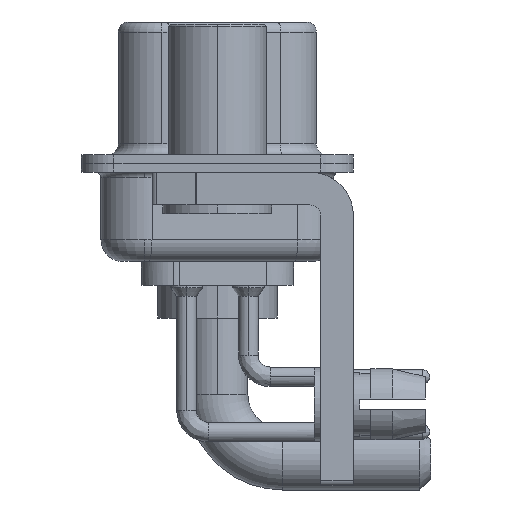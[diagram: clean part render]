
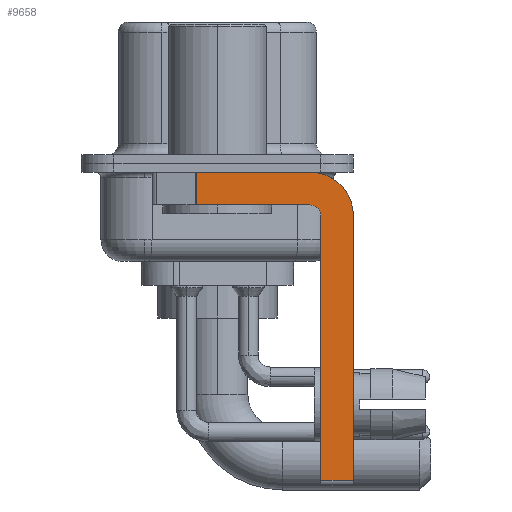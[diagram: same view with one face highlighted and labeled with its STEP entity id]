
A CAD part, left-side view. The second image highlights one B-rep face of the part: STEP entity #9658.
In plain terms, the highlighted planar face has unit normal (-1, 0, 0).
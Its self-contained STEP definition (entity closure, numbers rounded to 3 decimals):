
#695 = EDGE_LOOP ( 'NONE', ( #3606, #11332, #12984, #16502, #7405, #11200, #17029, #29080 ) ) ;
#768 = EDGE_CURVE ( 'NONE', #21767, #13116, #26312, .T. ) ;
#814 = DIRECTION ( 'NONE',  ( 0., 0., 1. ) ) ;
#1452 = VECTOR ( 'NONE', #12609, 1000. ) ;
#1464 = CARTESIAN_POINT ( 'NONE',  ( -2.9, 3., -0.4 ) ) ;
#2760 = DIRECTION ( 'NONE',  ( -1., 0., 0. ) ) ;
#2823 = CARTESIAN_POINT ( 'NONE',  ( -2.9, -4.25, -1.9 ) ) ;
#3297 = CARTESIAN_POINT ( 'NONE',  ( -2.9, 0.978, -1.9 ) ) ;
#3606 = ORIENTED_EDGE ( 'NONE', *, *, #768, .F. ) ;
#4051 = CIRCLE ( 'NONE', #5938, 2. ) ;
#4072 = CARTESIAN_POINT ( 'NONE',  ( -2.9, -4.75, -14.55 ) ) ;
#4102 = CARTESIAN_POINT ( 'NONE',  ( -2.9, -4.75, -14.8 ) ) ;
#4115 = EDGE_CURVE ( 'NONE', #13116, #25936, #4051, .T. ) ;
#4164 = EDGE_CURVE ( 'NONE', #28870, #18369, #13139, .T. ) ;
#4523 = CARTESIAN_POINT ( 'NONE',  ( -2.9, -4.25, -14.55 ) ) ;
#5938 = AXIS2_PLACEMENT_3D ( 'NONE', #18523, #11249, #20317 ) ;
#6212 = DIRECTION ( 'NONE',  ( 0., 0., -1. ) ) ;
#7405 = ORIENTED_EDGE ( 'NONE', *, *, #8785, .F. ) ;
#8454 = DIRECTION ( 'NONE',  ( 1., 0., 0. ) ) ;
#8785 = EDGE_CURVE ( 'NONE', #15551, #28870, #8856, .T. ) ;
#8856 = LINE ( 'NONE', #4102, #14145 ) ;
#9569 = CARTESIAN_POINT ( 'NONE',  ( -2.9, -4.75, -2.4 ) ) ;
#9650 = LINE ( 'NONE', #2823, #18186 ) ;
#9658 = ADVANCED_FACE ( 'NONE', ( #19751 ), #14989, .F. ) ;
#9834 = LINE ( 'NONE', #3297, #22312 ) ;
#10580 = CARTESIAN_POINT ( 'NONE',  ( -2.9, -6.25, -2.4 ) ) ;
#11200 = ORIENTED_EDGE ( 'NONE', *, *, #19081, .T. ) ;
#11249 = DIRECTION ( 'NONE',  ( 1., 0., 0. ) ) ;
#11332 = ORIENTED_EDGE ( 'NONE', *, *, #23194, .T. ) ;
#11954 = VECTOR ( 'NONE', #19138, 1000. ) ;
#12308 = LINE ( 'NONE', #23481, #11954 ) ;
#12609 = DIRECTION ( 'NONE',  ( 0., -1., 0. ) ) ;
#12887 = CARTESIAN_POINT ( 'NONE',  ( -2.9, 0.978, -1.9 ) ) ;
#12984 = ORIENTED_EDGE ( 'NONE', *, *, #14997, .F. ) ;
#13116 = VERTEX_POINT ( 'NONE', #16447 ) ;
#13139 = CIRCLE ( 'NONE', #20739, 0.5 ) ;
#14145 = VECTOR ( 'NONE', #17934, 1000. ) ;
#14989 = PLANE ( 'NONE',  #22765 ) ;
#14997 = EDGE_CURVE ( 'NONE', #18369, #16271, #9650, .T. ) ;
#15551 = VERTEX_POINT ( 'NONE', #4072 ) ;
#16271 = VERTEX_POINT ( 'NONE', #12887 ) ;
#16447 = CARTESIAN_POINT ( 'NONE',  ( -2.9, -4.25, -0.4 ) ) ;
#16502 = ORIENTED_EDGE ( 'NONE', *, *, #4164, .F. ) ;
#17029 = ORIENTED_EDGE ( 'NONE', *, *, #26976, .F. ) ;
#17083 = CARTESIAN_POINT ( 'NONE',  ( -2.9, -6.25, -14.55 ) ) ;
#17934 = DIRECTION ( 'NONE',  ( 0., 0., 1. ) ) ;
#18186 = VECTOR ( 'NONE', #22922, 1000. ) ;
#18245 = CARTESIAN_POINT ( 'NONE',  ( -2.9, -4.25, -1.9 ) ) ;
#18369 = VERTEX_POINT ( 'NONE', #18245 ) ;
#18523 = CARTESIAN_POINT ( 'NONE',  ( -2.9, -4.25, -2.4 ) ) ;
#18902 = DIRECTION ( 'NONE',  ( 0., 0., -1. ) ) ;
#19081 = EDGE_CURVE ( 'NONE', #15551, #25029, #28931, .T. ) ;
#19103 = CARTESIAN_POINT ( 'NONE',  ( -2.9, -4.25, -2.4 ) ) ;
#19138 = DIRECTION ( 'NONE',  ( 0., 0., -1. ) ) ;
#19606 = CARTESIAN_POINT ( 'NONE',  ( -2.9, -4.25, -2.4 ) ) ;
#19751 = FACE_OUTER_BOUND ( 'NONE', #695, .T. ) ;
#20317 = DIRECTION ( 'NONE',  ( 0., 0., -1. ) ) ;
#20739 = AXIS2_PLACEMENT_3D ( 'NONE', #19103, #2760, #814 ) ;
#21767 = VERTEX_POINT ( 'NONE', #25794 ) ;
#22312 = VECTOR ( 'NONE', #18902, 1000. ) ;
#22765 = AXIS2_PLACEMENT_3D ( 'NONE', #19606, #8454, #6212 ) ;
#22922 = DIRECTION ( 'NONE',  ( 0., 1., 0. ) ) ;
#23194 = EDGE_CURVE ( 'NONE', #21767, #16271, #9834, .T. ) ;
#23481 = CARTESIAN_POINT ( 'NONE',  ( -2.9, -6.25, -2.4 ) ) ;
#24622 = DIRECTION ( 'NONE',  ( 0., -1., 0. ) ) ;
#25029 = VERTEX_POINT ( 'NONE', #17083 ) ;
#25794 = CARTESIAN_POINT ( 'NONE',  ( -2.9, 0.978, -0.4 ) ) ;
#25936 = VERTEX_POINT ( 'NONE', #10580 ) ;
#26312 = LINE ( 'NONE', #1464, #1452 ) ;
#26976 = EDGE_CURVE ( 'NONE', #25936, #25029, #12308, .T. ) ;
#27328 = VECTOR ( 'NONE', #24622, 1000. ) ;
#28870 = VERTEX_POINT ( 'NONE', #9569 ) ;
#28931 = LINE ( 'NONE', #4523, #27328 ) ;
#29080 = ORIENTED_EDGE ( 'NONE', *, *, #4115, .F. ) ;
